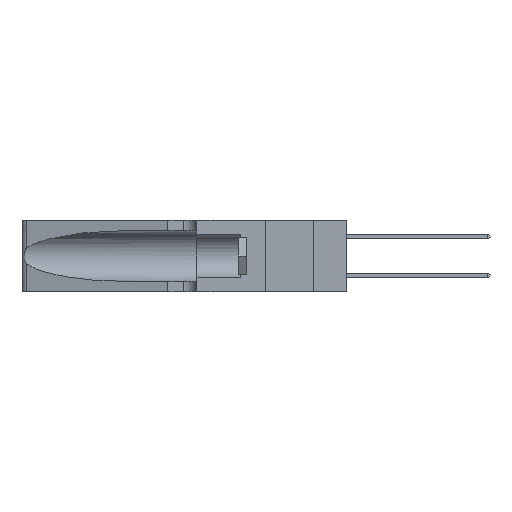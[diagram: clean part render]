
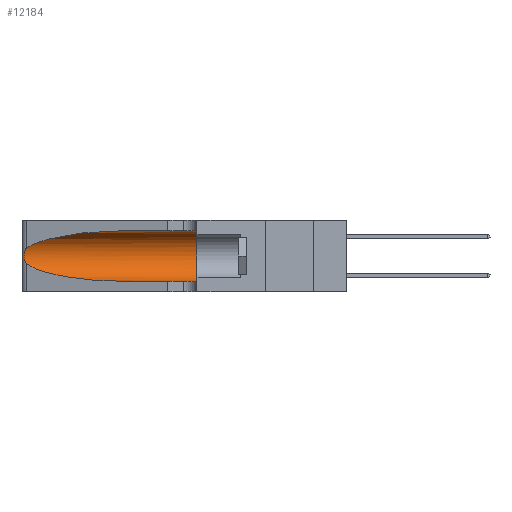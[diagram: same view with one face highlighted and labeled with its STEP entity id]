
A CAD part, left-side view. The second image highlights one B-rep face of the part: STEP entity #12184.
In plain terms, the highlighted cylindrical face has radius 3.308 mm (diameter 6.617 mm), a partial arc.
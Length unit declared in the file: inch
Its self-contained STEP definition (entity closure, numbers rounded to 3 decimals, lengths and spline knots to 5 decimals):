
#41 = CARTESIAN_POINT ( 'NONE',  ( 0.25639, 1.23186, 0.15144 ) ) ;
#482 = CARTESIAN_POINT ( 'NONE',  ( 0.2373, 1.15595, 0.08982 ) ) ;
#1721 =( BOUNDED_CURVE ( )  B_SPLINE_CURVE ( 3, ( #16902, #482, #5030, #3238 ),
 .UNSPECIFIED., .F., .T. ) 
 B_SPLINE_CURVE_WITH_KNOTS ( ( 4, 4 ),
 ( 3.44316, 4.71239 ),
 .UNSPECIFIED. ) 
 CURVE ( )  GEOMETRIC_REPRESENTATION_ITEM ( )  RATIONAL_B_SPLINE_CURVE ( ( 1., 0.87, 0.87, 1. ) ) 
 REPRESENTATION_ITEM ( '' )  );
#1830 = CARTESIAN_POINT ( 'NONE',  ( 0.1305, 1.61858, 0.05475 ) ) ;
#2399 = CARTESIAN_POINT ( 'NONE',  ( 0.25487, 1.22718, 0.14631 ) ) ;
#3238 = CARTESIAN_POINT ( 'NONE',  ( 0.1305, 0.72297, 0.05475 ) ) ;
#3271 = EDGE_CURVE ( 'NONE', #24636, #26921, #15713, .T. ) ;
#3471 = FACE_OUTER_BOUND ( 'NONE', #17367, .T. ) ;
#4280 = VECTOR ( 'NONE', #7812, 39.37008 ) ;
#4580 = CARTESIAN_POINT ( 'NONE',  ( 0.25639, 1.23184, 0.21858 ) ) ;
#4838 = B_SPLINE_CURVE_WITH_KNOTS ( 'NONE', 3,
 ( #15868, #15962, #4580, #20506, #6894, #22770, #9166, #25035, #11467, #27274, #13787, #41, #16059, #2399 ),
 .UNSPECIFIED., .F., .F.,
 ( 4, 2, 2, 2, 2, 2, 4 ),
 ( 0., 0.00027, 0.00053, 0.00107, 0.0016, 0.00187, 0.00214 ),
 .UNSPECIFIED. ) ;
#5030 = CARTESIAN_POINT ( 'NONE',  ( 0.18966, 0.96281, 0.05475 ) ) ;
#5299 = DIRECTION ( 'NONE',  ( 0., 0., -1. ) ) ;
#5348 = ORIENTED_EDGE ( 'NONE', *, *, #11832, .T. ) ;
#5524 = CARTESIAN_POINT ( 'NONE',  ( 0.1305, 1.61858, 0.31525 ) ) ;
#6591 = CARTESIAN_POINT ( 'NONE',  ( 0.1305, 0.35, 0.31525 ) ) ;
#6794 = CARTESIAN_POINT ( 'NONE',  ( 0.1305, 0.72297, 0.31525 ) ) ;
#6894 = CARTESIAN_POINT ( 'NONE',  ( 0.25854, 1.2359, 0.20912 ) ) ;
#7043 = CARTESIAN_POINT ( 'NONE',  ( 0.1305, 0.72297, 0.05475 ) ) ;
#7503 = CARTESIAN_POINT ( 'NONE',  ( 0.1305, 1.61858, 0.185 ) ) ;
#7693 = ORIENTED_EDGE ( 'NONE', *, *, #3271, .F. ) ;
#7812 = DIRECTION ( 'NONE',  ( 0., -1., 0. ) ) ;
#8239 = AXIS2_PLACEMENT_3D ( 'NONE', #7503, #18949, #5299 ) ;
#8801 = CYLINDRICAL_SURFACE ( 'NONE', #8239, 0.13025 ) ;
#9166 = CARTESIAN_POINT ( 'NONE',  ( 0.26075, 1.23896, 0.19203 ) ) ;
#9875 = CARTESIAN_POINT ( 'NONE',  ( 0.25487, 1.22718, 0.14631 ) ) ;
#10569 = EDGE_CURVE ( 'NONE', #24636, #14307, #24131, .T. ) ;
#11010 = DIRECTION ( 'NONE',  ( 0., -1., 0. ) ) ;
#11467 = CARTESIAN_POINT ( 'NONE',  ( 0.26017, 1.23833, 0.17102 ) ) ;
#11753 = DIRECTION ( 'NONE',  ( 0., 1., 0. ) ) ;
#11832 = EDGE_CURVE ( 'NONE', #23497, #22048, #18808, .T. ) ;
#12184 = ADVANCED_FACE ( 'NONE', ( #3471 ), #8801, .F. ) ;
#13787 = CARTESIAN_POINT ( 'NONE',  ( 0.25789, 1.23486, 0.15765 ) ) ;
#14307 = VERTEX_POINT ( 'NONE', #17741 ) ;
#15204 = CARTESIAN_POINT ( 'NONE',  ( 0.1305, 0.35, 0.05475 ) ) ;
#15713 = LINE ( 'NONE', #5524, #4280 ) ;
#15813 = ORIENTED_EDGE ( 'NONE', *, *, #28429, .T. ) ;
#15868 = CARTESIAN_POINT ( 'NONE',  ( 0.25487, 1.22718, 0.22369 ) ) ;
#15962 = CARTESIAN_POINT ( 'NONE',  ( 0.25555, 1.22994, 0.2215 ) ) ;
#16059 = CARTESIAN_POINT ( 'NONE',  ( 0.25555, 1.22993, 0.14849 ) ) ;
#16481 = CARTESIAN_POINT ( 'NONE',  ( 0.1305, 0.72297, 0.31525 ) ) ;
#16902 = CARTESIAN_POINT ( 'NONE',  ( 0.25487, 1.22718, 0.14631 ) ) ;
#17367 = EDGE_LOOP ( 'NONE', ( #24344, #15813, #26413, #5348, #29343, #7693 ) ) ;
#17741 = CARTESIAN_POINT ( 'NONE',  ( 0.25487, 1.22718, 0.22369 ) ) ;
#18101 = VECTOR ( 'NONE', #11010, 39.37008 ) ;
#18140 = CARTESIAN_POINT ( 'NONE',  ( 0.2373, 1.15595, 0.28018 ) ) ;
#18808 = LINE ( 'NONE', #1830, #18101 ) ;
#18949 = DIRECTION ( 'NONE',  ( 0., -1., 0. ) ) ;
#19027 = EDGE_CURVE ( 'NONE', #21005, #23497, #1721, .T. ) ;
#20420 = CARTESIAN_POINT ( 'NONE',  ( 0.18966, 0.96281, 0.31525 ) ) ;
#20506 = CARTESIAN_POINT ( 'NONE',  ( 0.25787, 1.23484, 0.2124 ) ) ;
#21005 = VERTEX_POINT ( 'NONE', #9875 ) ;
#22048 = VERTEX_POINT ( 'NONE', #15204 ) ;
#22672 = CARTESIAN_POINT ( 'NONE',  ( 0.25487, 1.22718, 0.22369 ) ) ;
#22770 = CARTESIAN_POINT ( 'NONE',  ( 0.26018, 1.23835, 0.19895 ) ) ;
#23497 = VERTEX_POINT ( 'NONE', #7043 ) ;
#24131 =( BOUNDED_CURVE ( )  B_SPLINE_CURVE ( 3, ( #6794, #20420, #18140, #22672 ),
 .UNSPECIFIED., .F., .F. ) 
 B_SPLINE_CURVE_WITH_KNOTS ( ( 4, 4 ),
 ( 1.5708, 2.84003 ),
 .UNSPECIFIED. ) 
 CURVE ( )  GEOMETRIC_REPRESENTATION_ITEM ( )  RATIONAL_B_SPLINE_CURVE ( ( 1., 0.87, 0.87, 1. ) ) 
 REPRESENTATION_ITEM ( '' )  );
#24344 = ORIENTED_EDGE ( 'NONE', *, *, #10569, .T. ) ;
#24636 = VERTEX_POINT ( 'NONE', #16481 ) ;
#25035 = CARTESIAN_POINT ( 'NONE',  ( 0.26075, 1.23896, 0.178 ) ) ;
#25195 = EDGE_CURVE ( 'NONE', #26921, #22048, #27504, .T. ) ;
#25319 = CARTESIAN_POINT ( 'NONE',  ( 0.1305, 0.35, 0.185 ) ) ;
#26413 = ORIENTED_EDGE ( 'NONE', *, *, #19027, .T. ) ;
#26921 = VERTEX_POINT ( 'NONE', #6591 ) ;
#27274 = CARTESIAN_POINT ( 'NONE',  ( 0.25856, 1.23593, 0.16098 ) ) ;
#27504 = CIRCLE ( 'NONE', #28535, 0.13025 ) ;
#27556 = DIRECTION ( 'NONE',  ( 0., 0., 1. ) ) ;
#28429 = EDGE_CURVE ( 'NONE', #14307, #21005, #4838, .T. ) ;
#28535 = AXIS2_PLACEMENT_3D ( 'NONE', #25319, #11753, #27556 ) ;
#29343 = ORIENTED_EDGE ( 'NONE', *, *, #25195, .F. ) ;
